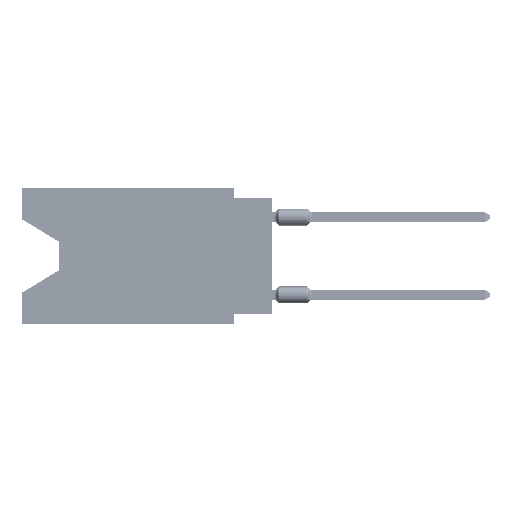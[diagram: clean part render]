
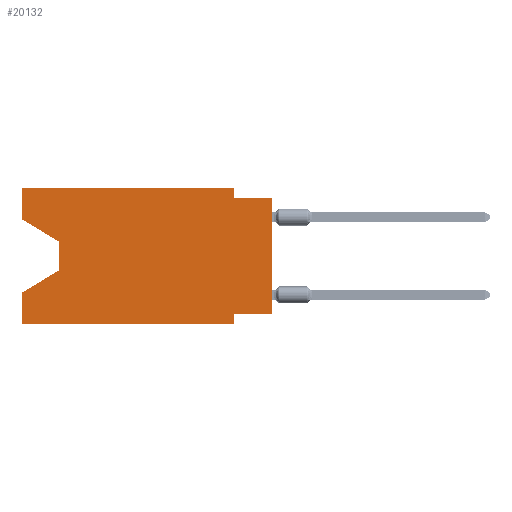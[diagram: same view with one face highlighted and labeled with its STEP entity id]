
A CAD part, left-side view. The second image highlights one B-rep face of the part: STEP entity #20132.
In plain terms, the highlighted planar face has unit normal (-1, 0, 0).
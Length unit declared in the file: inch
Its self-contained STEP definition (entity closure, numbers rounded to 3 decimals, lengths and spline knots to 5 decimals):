
#266 = VERTEX_POINT ( 'NONE', #43711 ) ;
#1758 = LINE ( 'NONE', #27192, #18068 ) ;
#2129 = DIRECTION ( 'NONE',  ( 1., 0., 0. ) ) ;
#3418 = ORIENTED_EDGE ( 'NONE', *, *, #37531, .F. ) ;
#3504 = EDGE_CURVE ( 'NONE', #76199, #92381, #76350, .T. ) ;
#5345 = VECTOR ( 'NONE', #46988, 39.37008 ) ;
#6265 = DIRECTION ( 'NONE',  ( 0., 0., -1. ) ) ;
#7667 = EDGE_CURVE ( 'NONE', #266, #41659, #32752, .T. ) ;
#8927 = VECTOR ( 'NONE', #98647, 39.37008 ) ;
#9163 = VECTOR ( 'NONE', #17127, 39.37008 ) ;
#9921 = CARTESIAN_POINT ( 'NONE',  ( 0., 0.645, 0. ) ) ;
#10072 = ORIENTED_EDGE ( 'NONE', *, *, #68892, .T. ) ;
#11622 = CARTESIAN_POINT ( 'NONE',  ( 0., 0., -0.325 ) ) ;
#13919 = CARTESIAN_POINT ( 'NONE',  ( 0., 0.55, -0.138 ) ) ;
#13988 = DIRECTION ( 'NONE',  ( 0., 0.855, -0.519 ) ) ;
#14951 = VERTEX_POINT ( 'NONE', #101125 ) ;
#15305 = DIRECTION ( 'NONE',  ( 0., -0.855, -0.519 ) ) ;
#16114 = LINE ( 'NONE', #65946, #8927 ) ;
#16727 = LINE ( 'NONE', #50470, #49347 ) ;
#17127 = DIRECTION ( 'NONE',  ( 0., 0., 1. ) ) ;
#18068 = VECTOR ( 'NONE', #105228, 39.37008 ) ;
#20132 = ADVANCED_FACE ( 'NONE', ( #76847 ), #94018, .F. ) ;
#21122 = CARTESIAN_POINT ( 'NONE',  ( 0., 0., -0.025 ) ) ;
#22153 = EDGE_LOOP ( 'NONE', ( #54768, #28975, #66254, #54721, #10072, #86817, #58524, #88439, #70875, #3418, #37143, #55667 ) ) ;
#22688 = EDGE_CURVE ( 'NONE', #92381, #55108, #1758, .T. ) ;
#23391 = CARTESIAN_POINT ( 'NONE',  ( 0., 0.55, -0.212 ) ) ;
#26087 = CARTESIAN_POINT ( 'NONE',  ( 0., 0., 0. ) ) ;
#27192 = CARTESIAN_POINT ( 'NONE',  ( 0., 0.645, 0. ) ) ;
#28874 = DIRECTION ( 'NONE',  ( 0., 0., -1. ) ) ;
#28975 = ORIENTED_EDGE ( 'NONE', *, *, #46473, .T. ) ;
#29203 = EDGE_CURVE ( 'NONE', #49074, #78613, #99223, .T. ) ;
#30303 = CARTESIAN_POINT ( 'NONE',  ( 0., 0., -0.025 ) ) ;
#32752 = LINE ( 'NONE', #26087, #57173 ) ;
#35315 = CARTESIAN_POINT ( 'NONE',  ( 0., 0.645, 0. ) ) ;
#35861 = DIRECTION ( 'NONE',  ( 0., 0., -1. ) ) ;
#36337 = DIRECTION ( 'NONE',  ( 0., 0., 1. ) ) ;
#36738 = CARTESIAN_POINT ( 'NONE',  ( 0., 0.1, -0.35 ) ) ;
#36855 = CARTESIAN_POINT ( 'NONE',  ( 0., 0.645, 0. ) ) ;
#37143 = ORIENTED_EDGE ( 'NONE', *, *, #22688, .F. ) ;
#37268 = CARTESIAN_POINT ( 'NONE',  ( 0., 0.645, 0. ) ) ;
#37531 = EDGE_CURVE ( 'NONE', #55108, #107364, #16727, .T. ) ;
#41659 = VERTEX_POINT ( 'NONE', #30303 ) ;
#43711 = CARTESIAN_POINT ( 'NONE',  ( 0., 0., -0.325 ) ) ;
#44359 = VECTOR ( 'NONE', #36337, 39.37008 ) ;
#45629 = CARTESIAN_POINT ( 'NONE',  ( 0., 0.645, -0.26975 ) ) ;
#46473 = EDGE_CURVE ( 'NONE', #81890, #49074, #91109, .T. ) ;
#46988 = DIRECTION ( 'NONE',  ( 0., 1., 0. ) ) ;
#49036 = LINE ( 'NONE', #57345, #94059 ) ;
#49074 = VERTEX_POINT ( 'NONE', #23391 ) ;
#49347 = VECTOR ( 'NONE', #6265, 39.37008 ) ;
#50470 = CARTESIAN_POINT ( 'NONE',  ( 0., 0.1, 0. ) ) ;
#51180 = DIRECTION ( 'NONE',  ( 0., 0., -1. ) ) ;
#53756 = LINE ( 'NONE', #61517, #90169 ) ;
#54721 = ORIENTED_EDGE ( 'NONE', *, *, #108107, .F. ) ;
#54768 = ORIENTED_EDGE ( 'NONE', *, *, #89260, .T. ) ;
#55108 = VERTEX_POINT ( 'NONE', #75654 ) ;
#55667 = ORIENTED_EDGE ( 'NONE', *, *, #3504, .F. ) ;
#57173 = VECTOR ( 'NONE', #58736, 39.37008 ) ;
#57345 = CARTESIAN_POINT ( 'NONE',  ( 0., 0.645, -0.08025 ) ) ;
#58214 = CARTESIAN_POINT ( 'NONE',  ( 0., 0.55, -0.212 ) ) ;
#58524 = ORIENTED_EDGE ( 'NONE', *, *, #85870, .F. ) ;
#58736 = DIRECTION ( 'NONE',  ( 0., 0., 1. ) ) ;
#61517 = CARTESIAN_POINT ( 'NONE',  ( 0., 0.1, -0.35 ) ) ;
#62885 = LINE ( 'NONE', #36855, #44359 ) ;
#63141 = CARTESIAN_POINT ( 'NONE',  ( 0., 0.1, -0.025 ) ) ;
#65946 = CARTESIAN_POINT ( 'NONE',  ( 0., 0.645, -0.35 ) ) ;
#66254 = ORIENTED_EDGE ( 'NONE', *, *, #29203, .T. ) ;
#68892 = EDGE_CURVE ( 'NONE', #79849, #83532, #16114, .T. ) ;
#70875 = ORIENTED_EDGE ( 'NONE', *, *, #76115, .F. ) ;
#75654 = CARTESIAN_POINT ( 'NONE',  ( 0., 0.1, 0. ) ) ;
#76115 = EDGE_CURVE ( 'NONE', #107364, #41659, #105814, .T. ) ;
#76199 = VERTEX_POINT ( 'NONE', #83628 ) ;
#76350 = LINE ( 'NONE', #9921, #9163 ) ;
#76847 = FACE_OUTER_BOUND ( 'NONE', #22153, .T. ) ;
#78613 = VERTEX_POINT ( 'NONE', #45629 ) ;
#79797 = DIRECTION ( 'NONE',  ( 0., -1., 0. ) ) ;
#79849 = VERTEX_POINT ( 'NONE', #90570 ) ;
#81890 = VERTEX_POINT ( 'NONE', #13919 ) ;
#82387 = VECTOR ( 'NONE', #13988, 39.37008 ) ;
#83532 = VERTEX_POINT ( 'NONE', #36738 ) ;
#83628 = CARTESIAN_POINT ( 'NONE',  ( 0., 0.645, -0.08025 ) ) ;
#85870 = EDGE_CURVE ( 'NONE', #266, #14951, #89093, .T. ) ;
#86583 = AXIS2_PLACEMENT_3D ( 'NONE', #35315, #2129, #35861 ) ;
#86817 = ORIENTED_EDGE ( 'NONE', *, *, #105540, .F. ) ;
#88439 = ORIENTED_EDGE ( 'NONE', *, *, #7667, .T. ) ;
#89093 = LINE ( 'NONE', #11622, #5345 ) ;
#89260 = EDGE_CURVE ( 'NONE', #76199, #81890, #49036, .T. ) ;
#90169 = VECTOR ( 'NONE', #28874, 39.37008 ) ;
#90570 = CARTESIAN_POINT ( 'NONE',  ( 0., 0.645, -0.35 ) ) ;
#90588 = VECTOR ( 'NONE', #51180, 39.37008 ) ;
#90951 = VECTOR ( 'NONE', #79797, 39.37008 ) ;
#91109 = LINE ( 'NONE', #100504, #90588 ) ;
#92381 = VERTEX_POINT ( 'NONE', #37268 ) ;
#94018 = PLANE ( 'NONE',  #86583 ) ;
#94059 = VECTOR ( 'NONE', #15305, 39.37008 ) ;
#98647 = DIRECTION ( 'NONE',  ( 0., -1., 0. ) ) ;
#99223 = LINE ( 'NONE', #58214, #82387 ) ;
#100504 = CARTESIAN_POINT ( 'NONE',  ( 0., 0.55, -0.138 ) ) ;
#101125 = CARTESIAN_POINT ( 'NONE',  ( 0., 0.1, -0.325 ) ) ;
#105228 = DIRECTION ( 'NONE',  ( 0., -1., 0. ) ) ;
#105540 = EDGE_CURVE ( 'NONE', #14951, #83532, #53756, .T. ) ;
#105814 = LINE ( 'NONE', #21122, #90951 ) ;
#107364 = VERTEX_POINT ( 'NONE', #63141 ) ;
#108107 = EDGE_CURVE ( 'NONE', #79849, #78613, #62885, .T. ) ;
